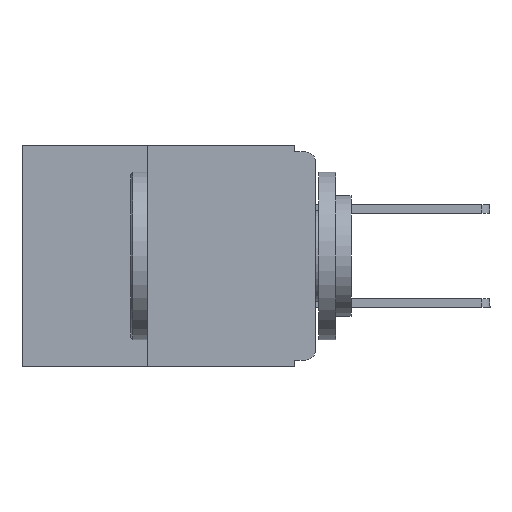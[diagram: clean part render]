
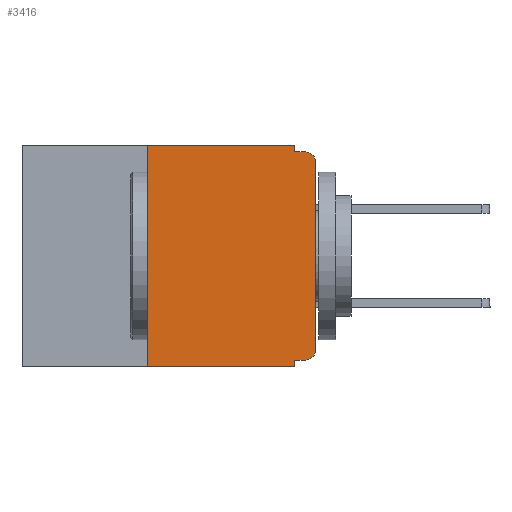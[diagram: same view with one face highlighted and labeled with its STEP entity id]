
A CAD part, left-side view. The second image highlights one B-rep face of the part: STEP entity #3416.
In plain terms, the highlighted planar face has unit normal (-1, 0, 0).
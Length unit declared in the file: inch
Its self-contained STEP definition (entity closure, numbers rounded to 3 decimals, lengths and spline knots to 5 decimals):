
#66 = FACE_OUTER_BOUND ( 'NONE', #1548, .T. ) ;
#185 = EDGE_CURVE ( 'NONE', #6916, #7400, #5699, .T. ) ;
#465 = EDGE_CURVE ( 'NONE', #6599, #2587, #10325, .T. ) ;
#475 = AXIS2_PLACEMENT_3D ( 'NONE', #11395, #11346, #11336 ) ;
#1060 = VERTEX_POINT ( 'NONE', #12221 ) ;
#1338 = CIRCLE ( 'NONE', #475, 0.015 ) ;
#1428 = CARTESIAN_POINT ( 'NONE',  ( 0., 0.031, -0.33 ) ) ;
#1548 = EDGE_LOOP ( 'NONE', ( #3608, #3899, #4086, #4142, #4158, #4316, #4380, #4470, #4621, #4884 ) ) ;
#1646 = EDGE_CURVE ( 'NONE', #1060, #10120, #11736, .T. ) ;
#1993 = VERTEX_POINT ( 'NONE', #9267 ) ;
#2178 = CARTESIAN_POINT ( 'NONE',  ( 0., 0.031, -0.33 ) ) ;
#2587 = VERTEX_POINT ( 'NONE', #1428 ) ;
#2728 = CIRCLE ( 'NONE', #11396, 0.015 ) ;
#2827 = CARTESIAN_POINT ( 'NONE',  ( 0., 0.25, -0.33 ) ) ;
#3416 = ADVANCED_FACE ( 'NONE', ( #66 ), #5409, .F. ) ;
#3608 = ORIENTED_EDGE ( 'NONE', *, *, #1646, .T. ) ;
#3899 = ORIENTED_EDGE ( 'NONE', *, *, #4969, .T. ) ;
#4086 = ORIENTED_EDGE ( 'NONE', *, *, #7300, .F. ) ;
#4142 = ORIENTED_EDGE ( 'NONE', *, *, #9663, .F. ) ;
#4158 = ORIENTED_EDGE ( 'NONE', *, *, #9170, .F. ) ;
#4316 = ORIENTED_EDGE ( 'NONE', *, *, #185, .F. ) ;
#4380 = ORIENTED_EDGE ( 'NONE', *, *, #13016, .T. ) ;
#4386 = VERTEX_POINT ( 'NONE', #9279 ) ;
#4470 = ORIENTED_EDGE ( 'NONE', *, *, #465, .F. ) ;
#4518 = EDGE_CURVE ( 'NONE', #4589, #1060, #2728, .T. ) ;
#4589 = VERTEX_POINT ( 'NONE', #10203 ) ;
#4621 = ORIENTED_EDGE ( 'NONE', *, *, #6475, .F. ) ;
#4884 = ORIENTED_EDGE ( 'NONE', *, *, #4518, .T. ) ;
#4969 = EDGE_CURVE ( 'NONE', #10120, #1993, #1338, .T. ) ;
#5012 = CARTESIAN_POINT ( 'NONE',  ( 0., 0., -0.025 ) ) ;
#5073 = DIRECTION ( 'NONE',  ( 0., 0., 1. ) ) ;
#5212 = DIRECTION ( 'NONE',  ( 1., 0., 0. ) ) ;
#5409 = PLANE ( 'NONE',  #11688 ) ;
#5646 = VECTOR ( 'NONE', #12907, 39.37008 ) ;
#5665 = LINE ( 'NONE', #12971, #5646 ) ;
#5681 = VECTOR ( 'NONE', #8763, 39.37008 ) ;
#5699 = LINE ( 'NONE', #6074, #5681 ) ;
#6074 = CARTESIAN_POINT ( 'NONE',  ( 0., 0.25, -0.33 ) ) ;
#6226 = CARTESIAN_POINT ( 'NONE',  ( 0., 0.437, 0. ) ) ;
#6475 = EDGE_CURVE ( 'NONE', #4589, #6599, #12646, .T. ) ;
#6599 = VERTEX_POINT ( 'NONE', #7671 ) ;
#6902 = CARTESIAN_POINT ( 'NONE',  ( 0., 0.25, 0. ) ) ;
#6916 = VERTEX_POINT ( 'NONE', #2827 ) ;
#7195 = VECTOR ( 'NONE', #12681, 39.37008 ) ;
#7249 = LINE ( 'NONE', #12966, #7195 ) ;
#7300 = EDGE_CURVE ( 'NONE', #11207, #1993, #11220, .T. ) ;
#7400 = VERTEX_POINT ( 'NONE', #6902 ) ;
#7671 = CARTESIAN_POINT ( 'NONE',  ( 0., 0.031, -0.32 ) ) ;
#7934 = CARTESIAN_POINT ( 'NONE',  ( 0., 0., 0. ) ) ;
#8409 = DIRECTION ( 'NONE',  ( 0., 0., -1. ) ) ;
#8428 = DIRECTION ( 'NONE',  ( -1., 0., 0. ) ) ;
#8460 = CARTESIAN_POINT ( 'NONE',  ( 0., 0.015, -0.305 ) ) ;
#8661 = DIRECTION ( 'NONE',  ( 0., 1., 0. ) ) ;
#8763 = DIRECTION ( 'NONE',  ( 0., 0., 1. ) ) ;
#8804 = CARTESIAN_POINT ( 'NONE',  ( 0., 0., -0.32 ) ) ;
#9170 = EDGE_CURVE ( 'NONE', #7400, #4386, #7249, .T. ) ;
#9267 = CARTESIAN_POINT ( 'NONE',  ( 0., 0.015, -0.01 ) ) ;
#9279 = CARTESIAN_POINT ( 'NONE',  ( 0., 0.031, 0. ) ) ;
#9547 = DIRECTION ( 'NONE',  ( 0., -1., 0. ) ) ;
#9663 = EDGE_CURVE ( 'NONE', #4386, #11207, #5665, .T. ) ;
#9769 = DIRECTION ( 'NONE',  ( 0., -1., 0. ) ) ;
#9828 = VECTOR ( 'NONE', #12187, 39.37008 ) ;
#9932 = VECTOR ( 'NONE', #9547, 39.37008 ) ;
#9960 = CARTESIAN_POINT ( 'NONE',  ( 0., 0., -0.01 ) ) ;
#10048 = CARTESIAN_POINT ( 'NONE',  ( 0., 0.437, -0.33 ) ) ;
#10120 = VERTEX_POINT ( 'NONE', #5012 ) ;
#10129 = LINE ( 'NONE', #10048, #9932 ) ;
#10203 = CARTESIAN_POINT ( 'NONE',  ( 0., 0.015, -0.32 ) ) ;
#10325 = LINE ( 'NONE', #2178, #9828 ) ;
#11140 = VECTOR ( 'NONE', #5073, 39.37008 ) ;
#11152 = VECTOR ( 'NONE', #9769, 39.37008 ) ;
#11207 = VERTEX_POINT ( 'NONE', #12533 ) ;
#11220 = LINE ( 'NONE', #9960, #11152 ) ;
#11336 = DIRECTION ( 'NONE',  ( 0., 0., -1. ) ) ;
#11346 = DIRECTION ( 'NONE',  ( -1., 0., 0. ) ) ;
#11395 = CARTESIAN_POINT ( 'NONE',  ( 0., 0.015, -0.025 ) ) ;
#11396 = AXIS2_PLACEMENT_3D ( 'NONE', #8460, #8428, #8409 ) ;
#11688 = AXIS2_PLACEMENT_3D ( 'NONE', #6226, #5212, #12176 ) ;
#11736 = LINE ( 'NONE', #7934, #11140 ) ;
#12176 = DIRECTION ( 'NONE',  ( 0., 0., -1. ) ) ;
#12187 = DIRECTION ( 'NONE',  ( 0., 0., -1. ) ) ;
#12221 = CARTESIAN_POINT ( 'NONE',  ( 0., 0., -0.305 ) ) ;
#12533 = CARTESIAN_POINT ( 'NONE',  ( 0., 0.031, -0.01 ) ) ;
#12646 = LINE ( 'NONE', #8804, #12655 ) ;
#12655 = VECTOR ( 'NONE', #8661, 39.37008 ) ;
#12681 = DIRECTION ( 'NONE',  ( 0., -1., 0. ) ) ;
#12907 = DIRECTION ( 'NONE',  ( 0., 0., -1. ) ) ;
#12966 = CARTESIAN_POINT ( 'NONE',  ( 0., 0.437, 0. ) ) ;
#12971 = CARTESIAN_POINT ( 'NONE',  ( 0., 0.031, 0. ) ) ;
#13016 = EDGE_CURVE ( 'NONE', #6916, #2587, #10129, .T. ) ;
